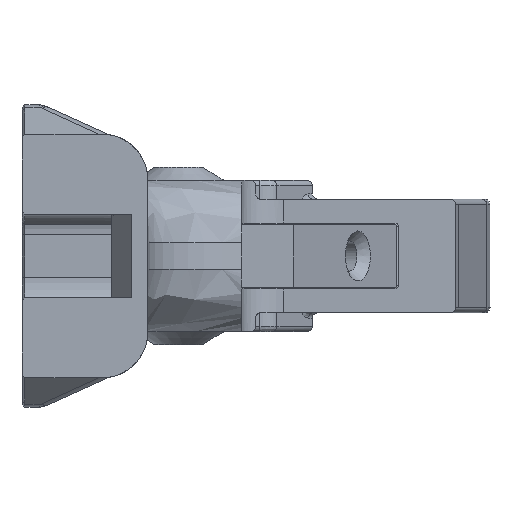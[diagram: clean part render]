
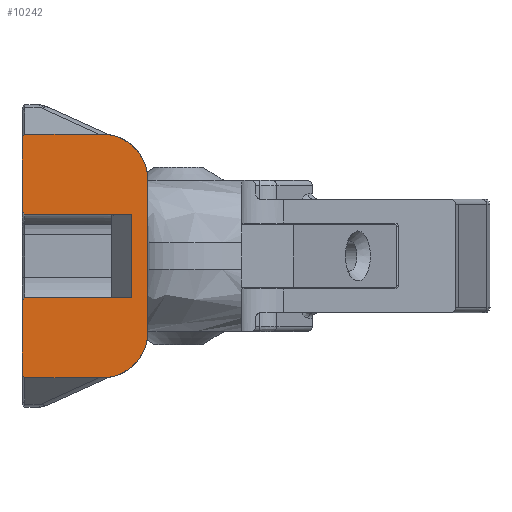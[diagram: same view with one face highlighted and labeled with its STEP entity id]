
A CAD part, left-side view. The second image highlights one B-rep face of the part: STEP entity #10242.
In plain terms, the highlighted planar face has unit normal (-1, 0, 0).
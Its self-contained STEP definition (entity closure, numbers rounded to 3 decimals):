
#87 = VERTEX_POINT ( 'NONE', #16583 ) ;
#157 = VERTEX_POINT ( 'NONE', #11360 ) ;
#290 = ORIENTED_EDGE ( 'NONE', *, *, #14820, .F. ) ;
#361 = DIRECTION ( 'NONE',  ( 0., -1., 0. ) ) ;
#423 = CARTESIAN_POINT ( 'NONE',  ( -193.873, 5.386, 7.55 ) ) ;
#633 = VERTEX_POINT ( 'NONE', #2889 ) ;
#642 = CARTESIAN_POINT ( 'NONE',  ( -193.873, 5.186, -17.567 ) ) ;
#697 = ORIENTED_EDGE ( 'NONE', *, *, #2796, .F. ) ;
#698 = VERTEX_POINT ( 'NONE', #3338 ) ;
#804 = CARTESIAN_POINT ( 'NONE',  ( -193.873, -6.534, -17.567 ) ) ;
#809 = LINE ( 'NONE', #3876, #7478 ) ;
#1004 = VERTEX_POINT ( 'NONE', #1505 ) ;
#1025 = VECTOR ( 'NONE', #8502, 1000. ) ;
#1369 = ORIENTED_EDGE ( 'NONE', *, *, #17104, .F. ) ;
#1398 = EDGE_CURVE ( 'NONE', #13406, #157, #10076, .T. ) ;
#1455 = VECTOR ( 'NONE', #15525, 1000. ) ;
#1499 = DIRECTION ( 'NONE',  ( 1., 0., 0. ) ) ;
#1505 = CARTESIAN_POINT ( 'NONE',  ( -193.873, 5.186, -5.35 ) ) ;
#1708 = CARTESIAN_POINT ( 'NONE',  ( -193.873, 5.186, 19.567 ) ) ;
#1769 = EDGE_CURVE ( 'NONE', #17303, #4000, #12826, .T. ) ;
#1813 = CARTESIAN_POINT ( 'NONE',  ( -193.873, -3.15, -5.35 ) ) ;
#1882 = VERTEX_POINT ( 'NONE', #12493 ) ;
#2170 = ORIENTED_EDGE ( 'NONE', *, *, #13689, .F. ) ;
#2652 = VECTOR ( 'NONE', #4408, 1000. ) ;
#2686 = DIRECTION ( 'NONE',  ( 0., 0.707, 0.707 ) ) ;
#2796 = EDGE_CURVE ( 'NONE', #16022, #11663, #16222, .T. ) ;
#2889 = CARTESIAN_POINT ( 'NONE',  ( -193.873, 5.186, 7.35 ) ) ;
#3335 = EDGE_CURVE ( 'NONE', #4326, #87, #8797, .T. ) ;
#3338 = CARTESIAN_POINT ( 'NONE',  ( -193.873, -11.114, 7.35 ) ) ;
#3605 = LINE ( 'NONE', #15460, #1025 ) ;
#3779 = AXIS2_PLACEMENT_3D ( 'NONE', #7783, #15815, #17207 ) ;
#3876 = CARTESIAN_POINT ( 'NONE',  ( -193.873, 5.586, -22.657 ) ) ;
#4000 = VERTEX_POINT ( 'NONE', #9835 ) ;
#4198 = CARTESIAN_POINT ( 'NONE',  ( -193.873, -13.591, 12.509 ) ) ;
#4326 = VERTEX_POINT ( 'NONE', #11199 ) ;
#4408 = DIRECTION ( 'NONE',  ( 0., -0.707, 0.707 ) ) ;
#4687 = ORIENTED_EDGE ( 'NONE', *, *, #1769, .F. ) ;
#4884 = DIRECTION ( 'NONE',  ( 0., 0., 1. ) ) ;
#4939 = VECTOR ( 'NONE', #2686, 1000. ) ;
#4991 = VERTEX_POINT ( 'NONE', #6286 ) ;
#5123 = VECTOR ( 'NONE', #16381, 1000. ) ;
#5272 = CARTESIAN_POINT ( 'NONE',  ( -193.873, -13.591, -10.511 ) ) ;
#5331 = VECTOR ( 'NONE', #14005, 1000. ) ;
#6085 = CARTESIAN_POINT ( 'NONE',  ( -193.873, 5.586, 19.167 ) ) ;
#6152 = LINE ( 'NONE', #6085, #1455 ) ;
#6286 = CARTESIAN_POINT ( 'NONE',  ( -193.873, -11.114, -5.35 ) ) ;
#6423 = EDGE_CURVE ( 'NONE', #1004, #4991, #11727, .T. ) ;
#6455 = EDGE_CURVE ( 'NONE', #633, #4326, #14473, .T. ) ;
#6643 = DIRECTION ( 'NONE',  ( 1., 0., 0. ) ) ;
#6739 = EDGE_CURVE ( 'NONE', #11663, #13406, #7535, .T. ) ;
#6935 = ORIENTED_EDGE ( 'NONE', *, *, #6739, .F. ) ;
#7218 = VECTOR ( 'NONE', #16694, 1000. ) ;
#7380 = ORIENTED_EDGE ( 'NONE', *, *, #3335, .F. ) ;
#7478 = VECTOR ( 'NONE', #9405, 1000. ) ;
#7535 = CIRCLE ( 'NONE', #8196, 7.057 ) ;
#7783 = CARTESIAN_POINT ( 'NONE',  ( -193.873, -3.15, -10.511 ) ) ;
#7902 = VECTOR ( 'NONE', #8435, 1000. ) ;
#8196 = AXIS2_PLACEMENT_3D ( 'NONE', #12040, #6643, #12218 ) ;
#8349 = LINE ( 'NONE', #16346, #7902 ) ;
#8435 = DIRECTION ( 'NONE',  ( 0., 1., 0. ) ) ;
#8502 = DIRECTION ( 'NONE',  ( 0., 1., 0. ) ) ;
#8797 = LINE ( 'NONE', #13176, #12830 ) ;
#9150 = EDGE_CURVE ( 'NONE', #4000, #1882, #809, .T. ) ;
#9173 = CIRCLE ( 'NONE', #15739, 7.057 ) ;
#9382 = EDGE_CURVE ( 'NONE', #698, #633, #3605, .T. ) ;
#9405 = DIRECTION ( 'NONE',  ( 0., 0., 1. ) ) ;
#9719 = CARTESIAN_POINT ( 'NONE',  ( -193.873, -6.534, -10.509 ) ) ;
#9729 = ORIENTED_EDGE ( 'NONE', *, *, #17450, .F. ) ;
#9835 = CARTESIAN_POINT ( 'NONE',  ( -193.873, 5.586, -17.167 ) ) ;
#10068 = EDGE_CURVE ( 'NONE', #87, #16022, #6152, .T. ) ;
#10076 = LINE ( 'NONE', #5272, #5123 ) ;
#10242 = ADVANCED_FACE ( 'NONE', ( #15136 ), #14677, .F. ) ;
#10613 = CARTESIAN_POINT ( 'NONE',  ( -193.873, -6.534, 19.567 ) ) ;
#11199 = CARTESIAN_POINT ( 'NONE',  ( -193.873, 5.586, 7.75 ) ) ;
#11244 = CARTESIAN_POINT ( 'NONE',  ( -193.873, 5.386, -5.55 ) ) ;
#11360 = CARTESIAN_POINT ( 'NONE',  ( -193.873, -13.591, -10.509 ) ) ;
#11593 = ORIENTED_EDGE ( 'NONE', *, *, #1398, .F. ) ;
#11663 = VERTEX_POINT ( 'NONE', #10613 ) ;
#11727 = LINE ( 'NONE', #1813, #12564 ) ;
#11738 = DIRECTION ( 'NONE',  ( 0., 0., 1. ) ) ;
#11890 = ORIENTED_EDGE ( 'NONE', *, *, #6455, .F. ) ;
#12040 = CARTESIAN_POINT ( 'NONE',  ( -193.873, -6.534, 12.509 ) ) ;
#12218 = DIRECTION ( 'NONE',  ( 0., -1., 0. ) ) ;
#12457 = DIRECTION ( 'NONE',  ( 0., -1., 0. ) ) ;
#12493 = CARTESIAN_POINT ( 'NONE',  ( -193.873, 5.586, -5.75 ) ) ;
#12564 = VECTOR ( 'NONE', #361, 1000. ) ;
#12826 = LINE ( 'NONE', #16052, #4939 ) ;
#12830 = VECTOR ( 'NONE', #4884, 1000. ) ;
#12990 = EDGE_LOOP ( 'NONE', ( #15529, #290, #15897, #4687, #2170, #1369, #11593, #6935, #697, #13175, #7380, #11890, #14286, #9729 ) ) ;
#13175 = ORIENTED_EDGE ( 'NONE', *, *, #10068, .F. ) ;
#13176 = CARTESIAN_POINT ( 'NONE',  ( -193.873, 5.586, -22.657 ) ) ;
#13406 = VERTEX_POINT ( 'NONE', #4198 ) ;
#13552 = LINE ( 'NONE', #11244, #2652 ) ;
#13689 = EDGE_CURVE ( 'NONE', #15556, #17303, #8349, .T. ) ;
#14005 = DIRECTION ( 'NONE',  ( 0., -1., 0. ) ) ;
#14251 = VECTOR ( 'NONE', #11738, 1000. ) ;
#14286 = ORIENTED_EDGE ( 'NONE', *, *, #9382, .F. ) ;
#14473 = LINE ( 'NONE', #423, #7218 ) ;
#14677 = PLANE ( 'NONE',  #3779 ) ;
#14820 = EDGE_CURVE ( 'NONE', #1882, #1004, #13552, .T. ) ;
#15136 = FACE_OUTER_BOUND ( 'NONE', #12990, .T. ) ;
#15428 = CARTESIAN_POINT ( 'NONE',  ( -193.873, -3.15, 19.567 ) ) ;
#15460 = CARTESIAN_POINT ( 'NONE',  ( -193.873, -3.15, 7.35 ) ) ;
#15525 = DIRECTION ( 'NONE',  ( 0., -0.707, 0.707 ) ) ;
#15527 = LINE ( 'NONE', #17587, #14251 ) ;
#15529 = ORIENTED_EDGE ( 'NONE', *, *, #6423, .F. ) ;
#15556 = VERTEX_POINT ( 'NONE', #804 ) ;
#15739 = AXIS2_PLACEMENT_3D ( 'NONE', #9719, #1499, #12457 ) ;
#15815 = DIRECTION ( 'NONE',  ( 1., 0., 0. ) ) ;
#15897 = ORIENTED_EDGE ( 'NONE', *, *, #9150, .F. ) ;
#16022 = VERTEX_POINT ( 'NONE', #1708 ) ;
#16052 = CARTESIAN_POINT ( 'NONE',  ( -193.873, 5.186, -17.567 ) ) ;
#16222 = LINE ( 'NONE', #15428, #5331 ) ;
#16346 = CARTESIAN_POINT ( 'NONE',  ( -193.873, -3.15, -17.567 ) ) ;
#16381 = DIRECTION ( 'NONE',  ( 0., 0., -1. ) ) ;
#16583 = CARTESIAN_POINT ( 'NONE',  ( -193.873, 5.586, 19.167 ) ) ;
#16694 = DIRECTION ( 'NONE',  ( 0., 0.707, 0.707 ) ) ;
#17104 = EDGE_CURVE ( 'NONE', #157, #15556, #9173, .T. ) ;
#17207 = DIRECTION ( 'NONE',  ( 0., 1., 0. ) ) ;
#17303 = VERTEX_POINT ( 'NONE', #642 ) ;
#17450 = EDGE_CURVE ( 'NONE', #4991, #698, #15527, .T. ) ;
#17587 = CARTESIAN_POINT ( 'NONE',  ( -193.873, -11.114, -10.511 ) ) ;
